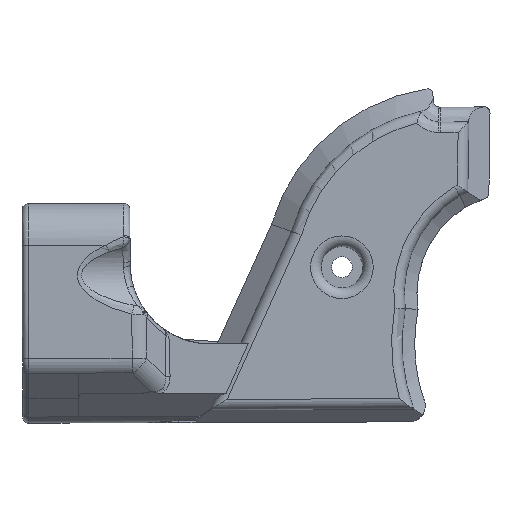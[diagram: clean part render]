
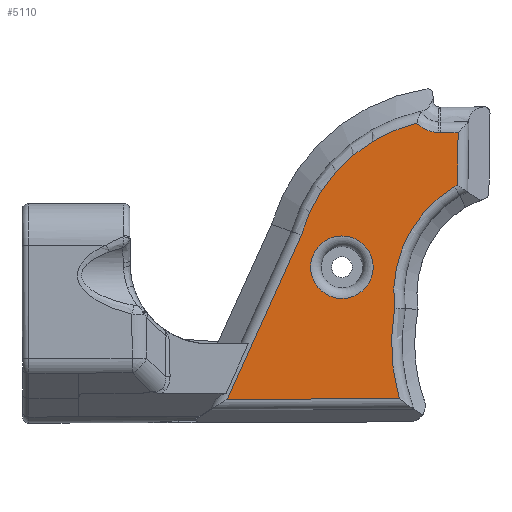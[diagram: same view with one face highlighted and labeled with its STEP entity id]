
A CAD part, left-side view. The second image highlights one B-rep face of the part: STEP entity #5110.
In plain terms, the highlighted planar face has unit normal (-1, 0, 0).
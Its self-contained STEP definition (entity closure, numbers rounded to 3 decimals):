
#98=FACE_BOUND('',#670,.T.);
#203=PLANE('',#5529);
#360=FACE_OUTER_BOUND('',#669,.T.);
#669=EDGE_LOOP('',(#3811,#3812,#3813,#3814,#3815,#3816,#3817,#3818,#3819,
#3820));
#670=EDGE_LOOP('',(#3821));
#952=CIRCLE('',#5526,7.54);
#955=CIRCLE('',#5530,38.544);
#956=CIRCLE('',#5531,47.886);
#957=CIRCLE('',#5532,30.086);
#1126=B_SPLINE_CURVE_WITH_KNOTS('',3,(#11129,#11130,#11131,#11132,#11133),
 .UNSPECIFIED.,.F.,.F.,(4,1,4),(-0.583,-0.335,0.),
 .UNSPECIFIED.);
#1388=LINE('',#10057,#1675);
#1506=LINE('',#11125,#1793);
#1507=LINE('',#11127,#1794);
#1508=LINE('',#11136,#1795);
#1509=LINE('',#11142,#1796);
#1510=LINE('',#11143,#1797);
#1675=VECTOR('',#5882,10.);
#1793=VECTOR('',#6358,10.);
#1794=VECTOR('',#6359,10.);
#1795=VECTOR('',#6362,10.);
#1796=VECTOR('',#6367,10.);
#1797=VECTOR('',#6368,10.);
#1998=VERTEX_POINT('',#10054);
#1999=VERTEX_POINT('',#10056);
#2161=VERTEX_POINT('',#11117);
#2163=VERTEX_POINT('',#11123);
#2164=VERTEX_POINT('',#11124);
#2165=VERTEX_POINT('',#11126);
#2166=VERTEX_POINT('',#11128);
#2167=VERTEX_POINT('',#11135);
#2168=VERTEX_POINT('',#11137);
#2169=VERTEX_POINT('',#11139);
#2170=VERTEX_POINT('',#11141);
#2527=EDGE_CURVE('',#1998,#1999,#1388,.T.);
#2776=EDGE_CURVE('',#2161,#2161,#952,.T.);
#2779=EDGE_CURVE('',#2163,#2164,#1506,.T.);
#2780=EDGE_CURVE('',#2165,#2163,#1507,.T.);
#2781=EDGE_CURVE('',#2166,#2165,#1126,.T.);
#2782=EDGE_CURVE('',#1999,#2166,#955,.T.);
#2783=EDGE_CURVE('',#2167,#1998,#1508,.T.);
#2784=EDGE_CURVE('',#2168,#2167,#956,.T.);
#2785=EDGE_CURVE('',#2169,#2168,#957,.T.);
#2786=EDGE_CURVE('',#2170,#2169,#1509,.T.);
#2787=EDGE_CURVE('',#2164,#2170,#1510,.T.);
#3811=ORIENTED_EDGE('',*,*,#2779,.F.);
#3812=ORIENTED_EDGE('',*,*,#2780,.F.);
#3813=ORIENTED_EDGE('',*,*,#2781,.F.);
#3814=ORIENTED_EDGE('',*,*,#2782,.F.);
#3815=ORIENTED_EDGE('',*,*,#2527,.F.);
#3816=ORIENTED_EDGE('',*,*,#2783,.F.);
#3817=ORIENTED_EDGE('',*,*,#2784,.F.);
#3818=ORIENTED_EDGE('',*,*,#2785,.F.);
#3819=ORIENTED_EDGE('',*,*,#2786,.F.);
#3820=ORIENTED_EDGE('',*,*,#2787,.F.);
#3821=ORIENTED_EDGE('',*,*,#2776,.F.);
#5110=ADVANCED_FACE('',(#360,#98),#203,.F.);
#5526=AXIS2_PLACEMENT_3D('',#11118,#6350,#6351);
#5529=AXIS2_PLACEMENT_3D('',#11122,#6356,#6357);
#5530=AXIS2_PLACEMENT_3D('',#11134,#6360,#6361);
#5531=AXIS2_PLACEMENT_3D('',#11138,#6363,#6364);
#5532=AXIS2_PLACEMENT_3D('',#11140,#6365,#6366);
#5882=DIRECTION('',(0.,-0.412,0.911));
#6350=DIRECTION('center_axis',(-1.,0.,0.));
#6351=DIRECTION('ref_axis',(0.,0.,
-1.));
#6356=DIRECTION('center_axis',(1.,0.,0.));
#6357=DIRECTION('ref_axis',(0.,1.,0.026));
#6358=DIRECTION('',(0.,-1.,0.005));
#6359=DIRECTION('',(0.,-1.,-0.026));
#6360=DIRECTION('center_axis',(1.,0.,0.));
#6361=DIRECTION('ref_axis',(0.,0.68,0.733));
#6362=DIRECTION('',(0.,1.,-0.003));
#6363=DIRECTION('center_axis',(-1.,0.,0.));
#6364=DIRECTION('ref_axis',(0.,0.996,-0.086));
#6365=DIRECTION('center_axis',(-1.,0.,0.));
#6366=DIRECTION('ref_axis',(0.,0.901,0.434));
#6367=DIRECTION('',(0.,0.915,-0.405));
#6368=DIRECTION('',(0.,0.014,-1.));
#10054=CARTESIAN_POINT('',(14.533,-25.748,-0.124));
#10056=CARTESIAN_POINT('',(14.533,-43.628,39.412));
#10057=CARTESIAN_POINT('',(14.533,-43.457,39.036));
#11117=CARTESIAN_POINT('',(14.533,-53.413,39.241));
#11118=CARTESIAN_POINT('Origin',(14.533,-53.413,31.701));
#11122=CARTESIAN_POINT('Origin',(14.533,-53.402,34.294));
#11123=CARTESIAN_POINT('',(14.533,-77.181,64.134));
#11124=CARTESIAN_POINT('',(14.533,-81.411,64.154));
#11125=CARTESIAN_POINT('',(14.533,-68.632,64.095));
#11126=CARTESIAN_POINT('',(14.533,-76.656,64.148));
#11127=CARTESIAN_POINT('',(14.533,-65.67,64.435));
#11128=CARTESIAN_POINT('',(14.533,-71.439,66.408));
#11129=CARTESIAN_POINT('Ctrl Pts',(14.533,-71.441,66.41));
#11130=CARTESIAN_POINT('Ctrl Pts',(14.533,-72.023,65.823));
#11131=CARTESIAN_POINT('Ctrl Pts',(14.533,-73.61,64.661));
#11132=CARTESIAN_POINT('Ctrl Pts',(14.533,-75.541,64.177));
#11133=CARTESIAN_POINT('Ctrl Pts',(14.533,-76.656,64.148));
#11134=CARTESIAN_POINT('Origin',(14.533,-80.74,29.003));
#11135=CARTESIAN_POINT('',(14.533,-67.252,0.016));
#11136=CARTESIAN_POINT('',(14.533,-37.657,-0.084));
#11137=CARTESIAN_POINT('',(14.533,-66.107,21.746));
#11138=CARTESIAN_POINT('Origin',(14.533,-113.248,13.336));
#11139=CARTESIAN_POINT('',(14.533,-80.617,51.162));
#11140=CARTESIAN_POINT('Origin',(14.533,-95.982,25.295));
#11141=CARTESIAN_POINT('',(14.533,-81.233,51.434));
#11142=CARTESIAN_POINT('',(14.533,-66.188,44.778));
#11143=CARTESIAN_POINT('',(14.533,-81.098,41.857));
